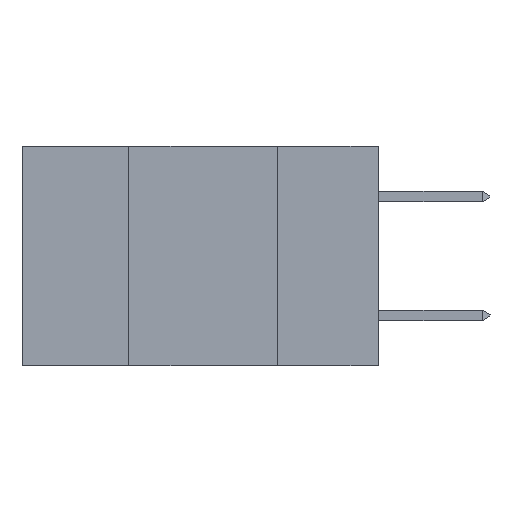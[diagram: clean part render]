
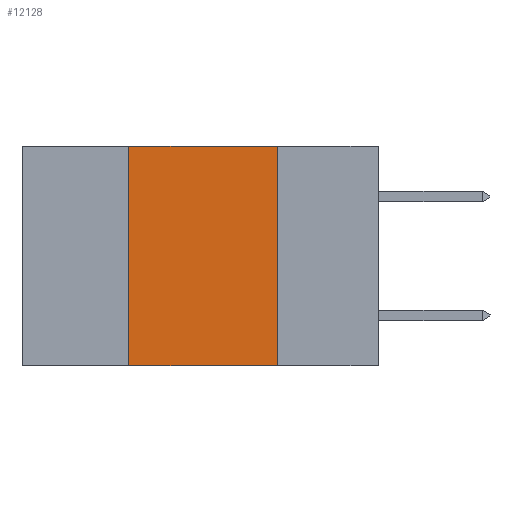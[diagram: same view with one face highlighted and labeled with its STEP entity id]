
A CAD part, left-side view. The second image highlights one B-rep face of the part: STEP entity #12128.
In plain terms, the highlighted planar face has unit normal (-1, 0, 0).
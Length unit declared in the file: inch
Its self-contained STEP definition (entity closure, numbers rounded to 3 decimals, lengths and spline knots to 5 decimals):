
#24 = DIRECTION ( 'NONE',  ( 0., -1., 0. ) ) ;
#725 = EDGE_CURVE ( 'NONE', #6158, #4359, #4972, .T. ) ;
#1339 = CARTESIAN_POINT ( 'NONE',  ( 0., 0.42, -0.37 ) ) ;
#1355 = VERTEX_POINT ( 'NONE', #20612 ) ;
#1746 = VECTOR ( 'NONE', #24, 39.37008 ) ;
#1950 = DIRECTION ( 'NONE',  ( 0., -1., 0. ) ) ;
#3198 = EDGE_LOOP ( 'NONE', ( #14309, #9400, #13727, #22881 ) ) ;
#4221 = DIRECTION ( 'NONE',  ( 0., 0., -1. ) ) ;
#4359 = VERTEX_POINT ( 'NONE', #22783 ) ;
#4972 = LINE ( 'NONE', #1339, #14191 ) ;
#5670 = CARTESIAN_POINT ( 'NONE',  ( 0., 0.17, 0. ) ) ;
#6158 = VERTEX_POINT ( 'NONE', #12435 ) ;
#7651 = VECTOR ( 'NONE', #20977, 39.37008 ) ;
#7656 = AXIS2_PLACEMENT_3D ( 'NONE', #17014, #15238, #4221 ) ;
#9400 = ORIENTED_EDGE ( 'NONE', *, *, #15268, .F. ) ;
#9672 = LINE ( 'NONE', #12954, #19467 ) ;
#12128 = ADVANCED_FACE ( 'NONE', ( #19300 ), #13415, .F. ) ;
#12435 = CARTESIAN_POINT ( 'NONE',  ( 0., 0.42, -0.37 ) ) ;
#12550 = LINE ( 'NONE', #15427, #7651 ) ;
#12954 = CARTESIAN_POINT ( 'NONE',  ( 0., 0.6, 0. ) ) ;
#13415 = PLANE ( 'NONE',  #7656 ) ;
#13727 = ORIENTED_EDGE ( 'NONE', *, *, #725, .F. ) ;
#14191 = VECTOR ( 'NONE', #15031, 39.37008 ) ;
#14309 = ORIENTED_EDGE ( 'NONE', *, *, #15565, .F. ) ;
#15031 = DIRECTION ( 'NONE',  ( 0., 0., 1. ) ) ;
#15238 = DIRECTION ( 'NONE',  ( 1., 0., 0. ) ) ;
#15268 = EDGE_CURVE ( 'NONE', #4359, #18071, #9672, .T. ) ;
#15427 = CARTESIAN_POINT ( 'NONE',  ( 0., 0.17, -0.37 ) ) ;
#15565 = EDGE_CURVE ( 'NONE', #18071, #1355, #12550, .T. ) ;
#17014 = CARTESIAN_POINT ( 'NONE',  ( 0., 0.6, 0. ) ) ;
#17448 = EDGE_CURVE ( 'NONE', #6158, #1355, #21296, .T. ) ;
#18071 = VERTEX_POINT ( 'NONE', #5670 ) ;
#19300 = FACE_OUTER_BOUND ( 'NONE', #3198, .T. ) ;
#19467 = VECTOR ( 'NONE', #1950, 39.37008 ) ;
#20612 = CARTESIAN_POINT ( 'NONE',  ( 0., 0.17, -0.37 ) ) ;
#20977 = DIRECTION ( 'NONE',  ( 0., 0., -1. ) ) ;
#21296 = LINE ( 'NONE', #21990, #1746 ) ;
#21990 = CARTESIAN_POINT ( 'NONE',  ( 0., 0.6, -0.37 ) ) ;
#22783 = CARTESIAN_POINT ( 'NONE',  ( 0., 0.42, 0. ) ) ;
#22881 = ORIENTED_EDGE ( 'NONE', *, *, #17448, .T. ) ;
